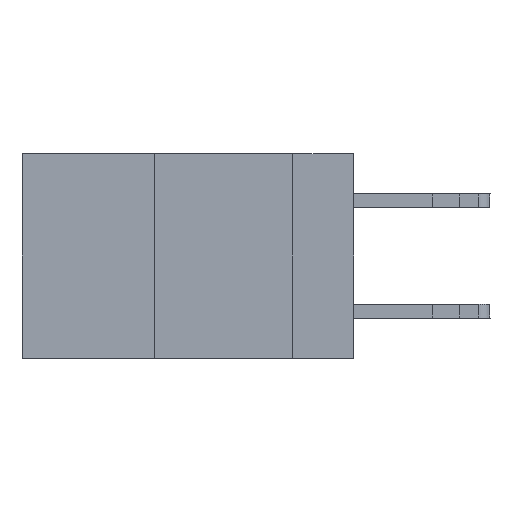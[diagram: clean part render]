
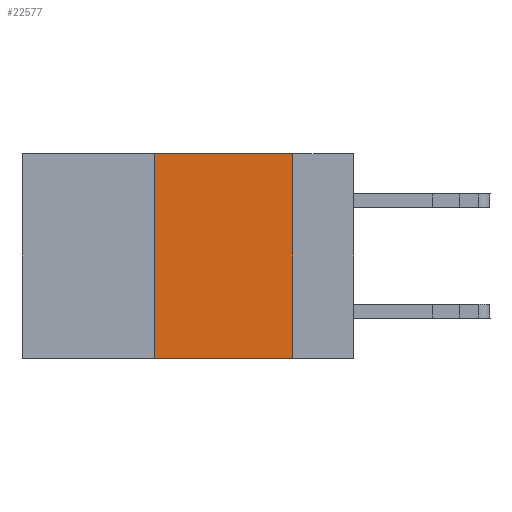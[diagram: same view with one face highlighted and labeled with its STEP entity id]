
A CAD part, left-side view. The second image highlights one B-rep face of the part: STEP entity #22577.
In plain terms, the highlighted planar face has unit normal (-1, 0, 0).
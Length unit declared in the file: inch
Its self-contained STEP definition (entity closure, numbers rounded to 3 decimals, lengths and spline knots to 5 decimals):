
#2222 = VECTOR ( 'NONE', #16376, 39.37008 ) ;
#2751 = CARTESIAN_POINT ( 'NONE',  ( 0., 0.36, 0. ) ) ;
#3058 = ORIENTED_EDGE ( 'NONE', *, *, #15372, .F. ) ;
#3384 = VERTEX_POINT ( 'NONE', #10407 ) ;
#3548 = PLANE ( 'NONE',  #11492 ) ;
#3967 = ORIENTED_EDGE ( 'NONE', *, *, #24014, .T. ) ;
#4154 = DIRECTION ( 'NONE',  ( 0., -1., 0. ) ) ;
#5190 = EDGE_CURVE ( 'NONE', #7982, #12122, #15430, .T. ) ;
#5387 = DIRECTION ( 'NONE',  ( 1., 0., 0. ) ) ;
#6063 = EDGE_LOOP ( 'NONE', ( #3058, #6253, #12909, #3967 ) ) ;
#6253 = ORIENTED_EDGE ( 'NONE', *, *, #5190, .F. ) ;
#6269 = LINE ( 'NONE', #8723, #2222 ) ;
#6848 = VECTOR ( 'NONE', #4154, 39.37008 ) ;
#7233 = CARTESIAN_POINT ( 'NONE',  ( 0., 0.6, 0. ) ) ;
#7737 = CARTESIAN_POINT ( 'NONE',  ( 0., 0.6, -0.37 ) ) ;
#7982 = VERTEX_POINT ( 'NONE', #2751 ) ;
#8438 = VERTEX_POINT ( 'NONE', #8737 ) ;
#8714 = FACE_OUTER_BOUND ( 'NONE', #6063, .T. ) ;
#8723 = CARTESIAN_POINT ( 'NONE',  ( 0., 0.11, 0. ) ) ;
#8737 = CARTESIAN_POINT ( 'NONE',  ( 0., 0.11, -0.37 ) ) ;
#9196 = DIRECTION ( 'NONE',  ( 0., 0., -1. ) ) ;
#10407 = CARTESIAN_POINT ( 'NONE',  ( 0., 0.36, -0.37 ) ) ;
#11492 = AXIS2_PLACEMENT_3D ( 'NONE', #7233, #5387, #9196 ) ;
#12122 = VERTEX_POINT ( 'NONE', #19773 ) ;
#12909 = ORIENTED_EDGE ( 'NONE', *, *, #18612, .F. ) ;
#13650 = CARTESIAN_POINT ( 'NONE',  ( 0., 0.36, 0. ) ) ;
#13881 = VECTOR ( 'NONE', #20844, 39.37008 ) ;
#15372 = EDGE_CURVE ( 'NONE', #12122, #8438, #6269, .T. ) ;
#15430 = LINE ( 'NONE', #17042, #13881 ) ;
#15498 = LINE ( 'NONE', #7737, #6848 ) ;
#16376 = DIRECTION ( 'NONE',  ( 0., 0., -1. ) ) ;
#17042 = CARTESIAN_POINT ( 'NONE',  ( 0., 0.6, 0. ) ) ;
#17306 = VECTOR ( 'NONE', #21398, 39.37008 ) ;
#18612 = EDGE_CURVE ( 'NONE', #3384, #7982, #23254, .T. ) ;
#19773 = CARTESIAN_POINT ( 'NONE',  ( 0., 0.11, 0. ) ) ;
#20844 = DIRECTION ( 'NONE',  ( 0., -1., 0. ) ) ;
#21398 = DIRECTION ( 'NONE',  ( 0., 0., 1. ) ) ;
#22577 = ADVANCED_FACE ( 'NONE', ( #8714 ), #3548, .F. ) ;
#23254 = LINE ( 'NONE', #13650, #17306 ) ;
#24014 = EDGE_CURVE ( 'NONE', #3384, #8438, #15498, .T. ) ;
